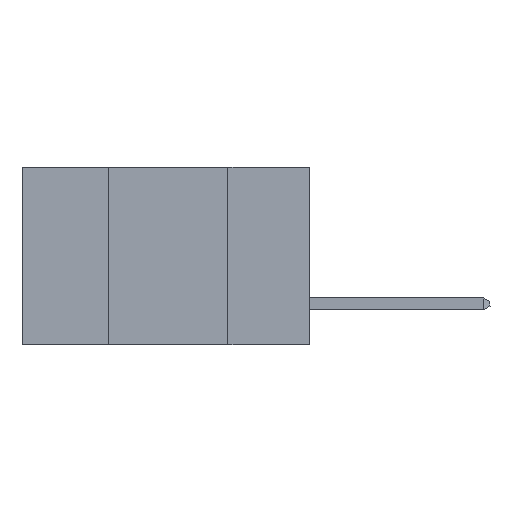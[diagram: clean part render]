
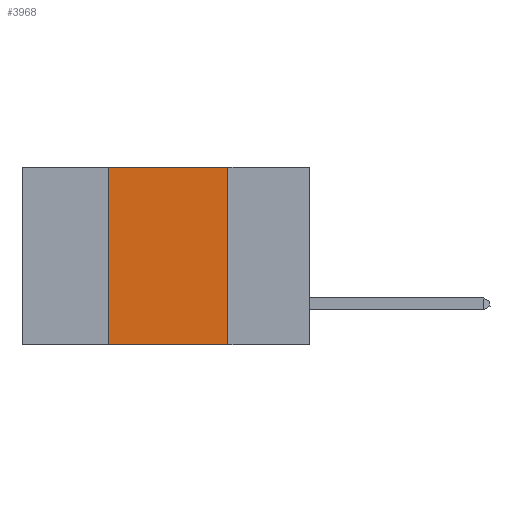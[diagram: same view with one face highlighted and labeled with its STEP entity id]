
A CAD part, left-side view. The second image highlights one B-rep face of the part: STEP entity #3968.
In plain terms, the highlighted planar face has unit normal (-1, 0, 0).
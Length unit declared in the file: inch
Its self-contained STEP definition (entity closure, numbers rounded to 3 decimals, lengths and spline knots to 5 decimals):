
#127 = CARTESIAN_POINT ( 'NONE',  ( 0., 0.42, 0. ) ) ;
#493 = VECTOR ( 'NONE', #2514, 39.37008 ) ;
#812 = VERTEX_POINT ( 'NONE', #5074 ) ;
#893 = EDGE_CURVE ( 'NONE', #5150, #1471, #5539, .T. ) ;
#921 = EDGE_CURVE ( 'NONE', #812, #1153, #8884, .T. ) ;
#1153 = VERTEX_POINT ( 'NONE', #2605 ) ;
#1471 = VERTEX_POINT ( 'NONE', #8164 ) ;
#1756 = DIRECTION ( 'NONE',  ( 0., 0., -1. ) ) ;
#1798 = CARTESIAN_POINT ( 'NONE',  ( 0., 0.6, 0. ) ) ;
#1809 = PLANE ( 'NONE',  #4559 ) ;
#2082 = DIRECTION ( 'NONE',  ( 0., -1., 0. ) ) ;
#2152 = DIRECTION ( 'NONE',  ( 0., 0., 1. ) ) ;
#2437 = CARTESIAN_POINT ( 'NONE',  ( 0., 0.17, 0. ) ) ;
#2458 = LINE ( 'NONE', #2437, #493 ) ;
#2514 = DIRECTION ( 'NONE',  ( 0., 0., -1. ) ) ;
#2530 = LINE ( 'NONE', #7413, #7789 ) ;
#2605 = CARTESIAN_POINT ( 'NONE',  ( 0., 0.17, -0.37 ) ) ;
#3216 = DIRECTION ( 'NONE',  ( 1., 0., 0. ) ) ;
#3533 = ORIENTED_EDGE ( 'NONE', *, *, #4948, .F. ) ;
#3558 = FACE_OUTER_BOUND ( 'NONE', #4329, .T. ) ;
#3968 = ADVANCED_FACE ( 'NONE', ( #3558 ), #1809, .F. ) ;
#4329 = EDGE_LOOP ( 'NONE', ( #3533, #6646, #7064, #7610 ) ) ;
#4559 = AXIS2_PLACEMENT_3D ( 'NONE', #1798, #3216, #1756 ) ;
#4948 = EDGE_CURVE ( 'NONE', #1471, #1153, #2458, .T. ) ;
#5074 = CARTESIAN_POINT ( 'NONE',  ( 0., 0.42, -0.37 ) ) ;
#5141 = VECTOR ( 'NONE', #2082, 39.37008 ) ;
#5150 = VERTEX_POINT ( 'NONE', #127 ) ;
#5338 = VECTOR ( 'NONE', #7217, 39.37008 ) ;
#5539 = LINE ( 'NONE', #8649, #5338 ) ;
#6646 = ORIENTED_EDGE ( 'NONE', *, *, #893, .F. ) ;
#6794 = EDGE_CURVE ( 'NONE', #812, #5150, #2530, .T. ) ;
#7064 = ORIENTED_EDGE ( 'NONE', *, *, #6794, .F. ) ;
#7217 = DIRECTION ( 'NONE',  ( 0., -1., 0. ) ) ;
#7413 = CARTESIAN_POINT ( 'NONE',  ( 0., 0.42, 0. ) ) ;
#7610 = ORIENTED_EDGE ( 'NONE', *, *, #921, .T. ) ;
#7789 = VECTOR ( 'NONE', #2152, 39.37008 ) ;
#8164 = CARTESIAN_POINT ( 'NONE',  ( 0., 0.17, 0. ) ) ;
#8567 = CARTESIAN_POINT ( 'NONE',  ( 0., 0.6, -0.37 ) ) ;
#8649 = CARTESIAN_POINT ( 'NONE',  ( 0., 0.6, 0. ) ) ;
#8884 = LINE ( 'NONE', #8567, #5141 ) ;
